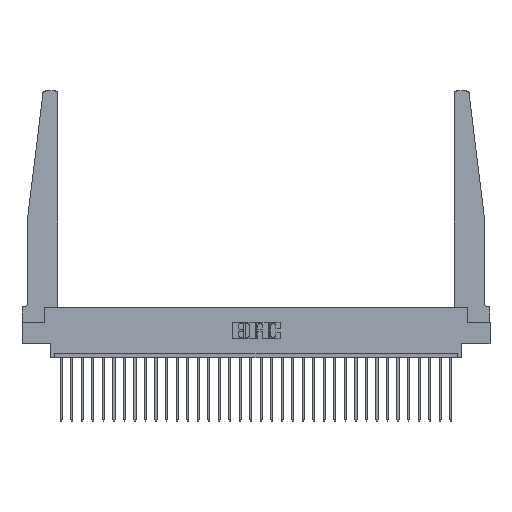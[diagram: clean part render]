
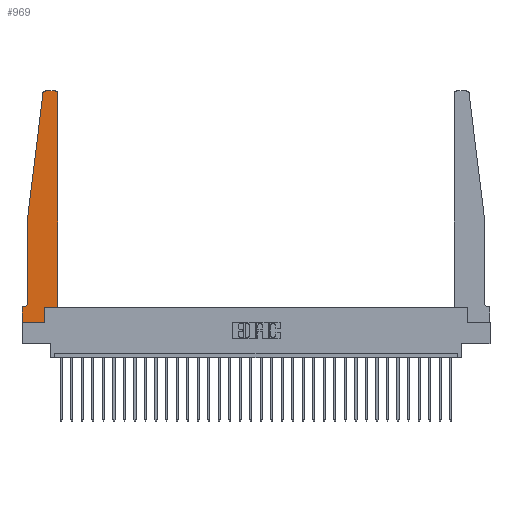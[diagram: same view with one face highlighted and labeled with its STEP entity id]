
A CAD part, top view. The second image highlights one B-rep face of the part: STEP entity #969.
In plain terms, the highlighted planar face has unit normal (0, 0, 1).
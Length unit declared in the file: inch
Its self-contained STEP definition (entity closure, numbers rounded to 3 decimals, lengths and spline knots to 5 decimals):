
#264 = CARTESIAN_POINT ( 'NONE',  ( 0.2605, 0.18, 0.37 ) ) ;
#425 = VERTEX_POINT ( 'NONE', #16305 ) ;
#964 = VERTEX_POINT ( 'NONE', #264 ) ;
#969 = ADVANCED_FACE ( 'NONE', ( #23051 ), #20812, .T. ) ;
#2031 = CARTESIAN_POINT ( 'NONE',  ( 0., 0., 0.37 ) ) ;
#2076 = VECTOR ( 'NONE', #22682, 39.37008 ) ;
#2241 = CARTESIAN_POINT ( 'NONE',  ( 0.25, 2.75, 0.37 ) ) ;
#2573 = CARTESIAN_POINT ( 'NONE',  ( 0., 0., 0.37 ) ) ;
#2873 = DIRECTION ( 'NONE',  ( 1., 0., 0. ) ) ;
#3211 = LINE ( 'NONE', #26871, #27577 ) ;
#3514 = EDGE_CURVE ( 'NONE', #964, #4103, #13889, .T. ) ;
#3629 = DIRECTION ( 'NONE',  ( 0., 0., 1. ) ) ;
#3760 = DIRECTION ( 'NONE',  ( 1., 0., 0. ) ) ;
#3942 = VERTEX_POINT ( 'NONE', #5101 ) ;
#4103 = VERTEX_POINT ( 'NONE', #22307 ) ;
#4237 = ORIENTED_EDGE ( 'NONE', *, *, #19553, .T. ) ;
#4640 = LINE ( 'NONE', #22781, #12308 ) ;
#4821 = LINE ( 'NONE', #2573, #8451 ) ;
#4916 = CARTESIAN_POINT ( 'NONE',  ( 0.425, 2.72, 0.37 ) ) ;
#5061 = DIRECTION ( 'NONE',  ( 1., 0., 0. ) ) ;
#5101 = CARTESIAN_POINT ( 'NONE',  ( 0.27653, 2.75, 0.37 ) ) ;
#5116 = DIRECTION ( 'NONE',  ( 0., -1., 0. ) ) ;
#5217 = ORIENTED_EDGE ( 'NONE', *, *, #20860, .T. ) ;
#6939 = CARTESIAN_POINT ( 'NONE',  ( 0., 0., 0.37 ) ) ;
#7130 = VECTOR ( 'NONE', #14291, 39.37008 ) ;
#7443 = DIRECTION ( 'NONE',  ( 0., 0., -1. ) ) ;
#7581 = CARTESIAN_POINT ( 'NONE',  ( 0.24675, 2.72367, 0.37 ) ) ;
#7769 = DIRECTION ( 'NONE',  ( 0., 0., 1. ) ) ;
#8451 = VECTOR ( 'NONE', #11629, 39.37008 ) ;
#8647 = ORIENTED_EDGE ( 'NONE', *, *, #14167, .T. ) ;
#8662 = CARTESIAN_POINT ( 'NONE',  ( 0.015, 0.1875, 0.37 ) ) ;
#8719 = EDGE_CURVE ( 'NONE', #19347, #20370, #24506, .T. ) ;
#9619 = CARTESIAN_POINT ( 'NONE',  ( 0.065, 0.2375, 0.37 ) ) ;
#10153 = CARTESIAN_POINT ( 'NONE',  ( 0.2605, 0.18, 0.37 ) ) ;
#10373 = VERTEX_POINT ( 'NONE', #22803 ) ;
#10510 = EDGE_CURVE ( 'NONE', #20370, #15004, #4821, .T. ) ;
#10536 = ORIENTED_EDGE ( 'NONE', *, *, #15618, .T. ) ;
#10881 = ORIENTED_EDGE ( 'NONE', *, *, #22244, .T. ) ;
#11096 = DIRECTION ( 'NONE',  ( 0., -1., 0. ) ) ;
#11629 = DIRECTION ( 'NONE',  ( 1., 0., 0. ) ) ;
#11680 = ORIENTED_EDGE ( 'NONE', *, *, #10510, .T. ) ;
#11874 = CARTESIAN_POINT ( 'NONE',  ( 0., 0.1875, 0.37 ) ) ;
#11911 = CARTESIAN_POINT ( 'NONE',  ( 0.015, 0.2375, 0.37 ) ) ;
#12193 = CARTESIAN_POINT ( 'NONE',  ( 0.425, 0.18, 0.37 ) ) ;
#12308 = VECTOR ( 'NONE', #20548, 39.37008 ) ;
#13333 = VECTOR ( 'NONE', #29049, 39.37008 ) ;
#13377 = LINE ( 'NONE', #2241, #13333 ) ;
#13407 = VECTOR ( 'NONE', #23667, 39.37008 ) ;
#13683 = EDGE_CURVE ( 'NONE', #3942, #19599, #28653, .T. ) ;
#13828 = VERTEX_POINT ( 'NONE', #8662 ) ;
#13889 = LINE ( 'NONE', #27476, #2076 ) ;
#14019 = VECTOR ( 'NONE', #11096, 39.37008 ) ;
#14167 = EDGE_CURVE ( 'NONE', #4103, #19998, #23526, .T. ) ;
#14276 = DIRECTION ( 'NONE',  ( -1., 0., 0. ) ) ;
#14291 = DIRECTION ( 'NONE',  ( 0., 1., 0. ) ) ;
#15004 = VERTEX_POINT ( 'NONE', #28344 ) ;
#15144 = ORIENTED_EDGE ( 'NONE', *, *, #3514, .T. ) ;
#15199 = CIRCLE ( 'NONE', #18046, 0.05 ) ;
#15618 = EDGE_CURVE ( 'NONE', #10373, #3942, #13377, .T. ) ;
#16305 = CARTESIAN_POINT ( 'NONE',  ( 0.065, 1.25, 0.37 ) ) ;
#16557 = EDGE_CURVE ( 'NONE', #425, #17662, #20866, .T. ) ;
#16874 = DIRECTION ( 'NONE',  ( -1., 0., 0. ) ) ;
#17662 = VERTEX_POINT ( 'NONE', #9619 ) ;
#18046 = AXIS2_PLACEMENT_3D ( 'NONE', #11911, #7443, #14276 ) ;
#18919 = CARTESIAN_POINT ( 'NONE',  ( 0.27653, 2.72, 0.37 ) ) ;
#19347 = VERTEX_POINT ( 'NONE', #28781 ) ;
#19553 = EDGE_CURVE ( 'NONE', #19599, #425, #4640, .T. ) ;
#19599 = VERTEX_POINT ( 'NONE', #7581 ) ;
#19998 = VERTEX_POINT ( 'NONE', #4916 ) ;
#20370 = VERTEX_POINT ( 'NONE', #6939 ) ;
#20548 = DIRECTION ( 'NONE',  ( -0.122, -0.992, 0. ) ) ;
#20568 = EDGE_CURVE ( 'NONE', #13828, #19347, #3211, .T. ) ;
#20812 = PLANE ( 'NONE',  #27847 ) ;
#20860 = EDGE_CURVE ( 'NONE', #17662, #13828, #15199, .T. ) ;
#20866 = LINE ( 'NONE', #25791, #24076 ) ;
#21008 = LINE ( 'NONE', #10153, #7130 ) ;
#21427 = CIRCLE ( 'NONE', #24318, 0.03 ) ;
#22208 = ORIENTED_EDGE ( 'NONE', *, *, #20568, .T. ) ;
#22244 = EDGE_CURVE ( 'NONE', #19998, #10373, #21427, .T. ) ;
#22307 = CARTESIAN_POINT ( 'NONE',  ( 0.425, 0.18, 0.37 ) ) ;
#22682 = DIRECTION ( 'NONE',  ( 1., 0., 0. ) ) ;
#22781 = CARTESIAN_POINT ( 'NONE',  ( 0.065, 1.25, 0.37 ) ) ;
#22803 = CARTESIAN_POINT ( 'NONE',  ( 0.395, 2.75, 0.37 ) ) ;
#23051 = FACE_OUTER_BOUND ( 'NONE', #27810, .T. ) ;
#23517 = ORIENTED_EDGE ( 'NONE', *, *, #27874, .T. ) ;
#23526 = LINE ( 'NONE', #12193, #13407 ) ;
#23667 = DIRECTION ( 'NONE',  ( 0., 1., 0. ) ) ;
#23870 = CARTESIAN_POINT ( 'NONE',  ( 0.395, 2.72, 0.37 ) ) ;
#24076 = VECTOR ( 'NONE', #5116, 39.37008 ) ;
#24318 = AXIS2_PLACEMENT_3D ( 'NONE', #23870, #3629, #3760 ) ;
#24356 = AXIS2_PLACEMENT_3D ( 'NONE', #18919, #7769, #2873 ) ;
#24506 = LINE ( 'NONE', #2031, #14019 ) ;
#25443 = DIRECTION ( 'NONE',  ( 0., 0., 1. ) ) ;
#25791 = CARTESIAN_POINT ( 'NONE',  ( 0.065, 1.25, 0.37 ) ) ;
#26871 = CARTESIAN_POINT ( 'NONE',  ( 0.065, 0.1875, 0.37 ) ) ;
#27474 = ORIENTED_EDGE ( 'NONE', *, *, #13683, .T. ) ;
#27476 = CARTESIAN_POINT ( 'NONE',  ( 0.425, 0.18, 0.37 ) ) ;
#27577 = VECTOR ( 'NONE', #16874, 39.37008 ) ;
#27810 = EDGE_LOOP ( 'NONE', ( #10536, #27474, #4237, #27879, #5217, #22208, #29216, #11680, #23517, #15144, #8647, #10881 ) ) ;
#27847 = AXIS2_PLACEMENT_3D ( 'NONE', #11874, #25443, #5061 ) ;
#27874 = EDGE_CURVE ( 'NONE', #15004, #964, #21008, .T. ) ;
#27879 = ORIENTED_EDGE ( 'NONE', *, *, #16557, .T. ) ;
#28344 = CARTESIAN_POINT ( 'NONE',  ( 0.2605, 0., 0.37 ) ) ;
#28653 = CIRCLE ( 'NONE', #24356, 0.03 ) ;
#28781 = CARTESIAN_POINT ( 'NONE',  ( 0., 0.1875, 0.37 ) ) ;
#29049 = DIRECTION ( 'NONE',  ( -1., 0., 0. ) ) ;
#29216 = ORIENTED_EDGE ( 'NONE', *, *, #8719, .T. ) ;
